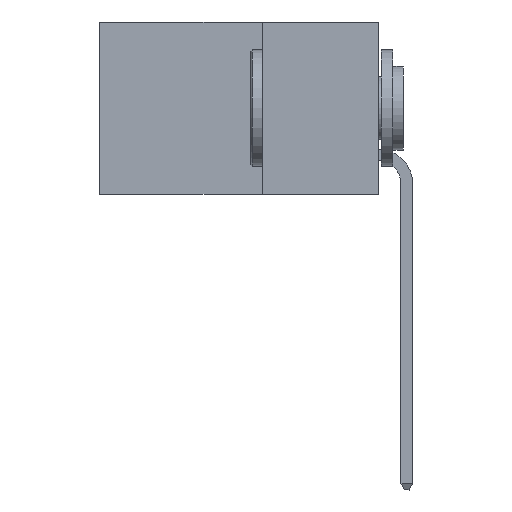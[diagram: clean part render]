
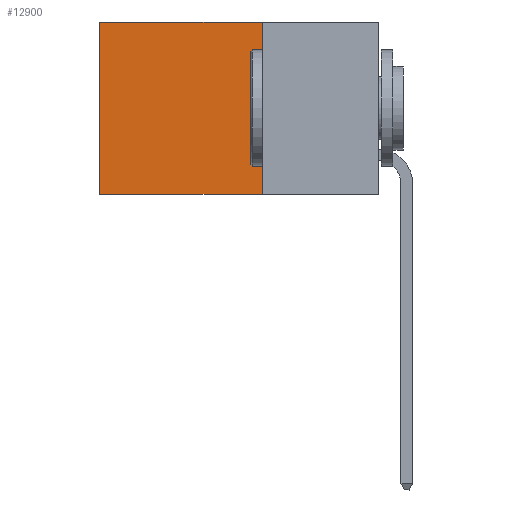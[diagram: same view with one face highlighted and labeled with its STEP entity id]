
A CAD part, left-side view. The second image highlights one B-rep face of the part: STEP entity #12900.
In plain terms, the highlighted planar face has unit normal (-1, 0, 0).
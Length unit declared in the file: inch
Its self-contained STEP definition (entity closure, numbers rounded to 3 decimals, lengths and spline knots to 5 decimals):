
#378 = CARTESIAN_POINT ( 'NONE',  ( 0.2615, 0.25, -0.37 ) ) ;
#1462 = VERTEX_POINT ( 'NONE', #378 ) ;
#1830 = CARTESIAN_POINT ( 'NONE',  ( 0.2615, 0.25, -0.37 ) ) ;
#1868 = DIRECTION ( 'NONE',  ( 0., 1., 0. ) ) ;
#2247 = VERTEX_POINT ( 'NONE', #4230 ) ;
#2530 = VECTOR ( 'NONE', #8465, 39.37008 ) ;
#2884 = AXIS2_PLACEMENT_3D ( 'NONE', #9756, #8778, #9684 ) ;
#3518 = VECTOR ( 'NONE', #1868, 39.37008 ) ;
#3574 = EDGE_LOOP ( 'NONE', ( #5027, #5815, #9888, #6665 ) ) ;
#4083 = LINE ( 'NONE', #1830, #8268 ) ;
#4184 = CARTESIAN_POINT ( 'NONE',  ( 0.2615, 0.25, -0.37 ) ) ;
#4230 = CARTESIAN_POINT ( 'NONE',  ( 0.2615, 0.25, 0. ) ) ;
#4293 = PLANE ( 'NONE',  #2884 ) ;
#5027 = ORIENTED_EDGE ( 'NONE', *, *, #8202, .T. ) ;
#5234 = LINE ( 'NONE', #4184, #2530 ) ;
#5314 = EDGE_CURVE ( 'NONE', #2247, #1462, #5234, .T. ) ;
#5768 = CARTESIAN_POINT ( 'NONE',  ( 0.2615, 0.6, -0.37 ) ) ;
#5794 = VERTEX_POINT ( 'NONE', #12613 ) ;
#5815 = ORIENTED_EDGE ( 'NONE', *, *, #12774, .F. ) ;
#6538 = VERTEX_POINT ( 'NONE', #9650 ) ;
#6665 = ORIENTED_EDGE ( 'NONE', *, *, #9199, .T. ) ;
#6854 = VECTOR ( 'NONE', #13293, 39.37008 ) ;
#8202 = EDGE_CURVE ( 'NONE', #5794, #6538, #11479, .T. ) ;
#8268 = VECTOR ( 'NONE', #10603, 39.37008 ) ;
#8465 = DIRECTION ( 'NONE',  ( 0., 0., -1. ) ) ;
#8778 = DIRECTION ( 'NONE',  ( 1., 0., 0. ) ) ;
#9199 = EDGE_CURVE ( 'NONE', #2247, #5794, #9446, .T. ) ;
#9446 = LINE ( 'NONE', #10508, #3518 ) ;
#9650 = CARTESIAN_POINT ( 'NONE',  ( 0.2615, 0.6, -0.37 ) ) ;
#9684 = DIRECTION ( 'NONE',  ( 0., 0., -1. ) ) ;
#9756 = CARTESIAN_POINT ( 'NONE',  ( 0.2615, 0.25, -0.37 ) ) ;
#9888 = ORIENTED_EDGE ( 'NONE', *, *, #5314, .F. ) ;
#9893 = FACE_OUTER_BOUND ( 'NONE', #3574, .T. ) ;
#10508 = CARTESIAN_POINT ( 'NONE',  ( 0.2615, 0.25, 0. ) ) ;
#10603 = DIRECTION ( 'NONE',  ( 0., 1., 0. ) ) ;
#11479 = LINE ( 'NONE', #5768, #6854 ) ;
#12613 = CARTESIAN_POINT ( 'NONE',  ( 0.2615, 0.6, 0. ) ) ;
#12774 = EDGE_CURVE ( 'NONE', #1462, #6538, #4083, .T. ) ;
#12900 = ADVANCED_FACE ( 'NONE', ( #9893 ), #4293, .F. ) ;
#13293 = DIRECTION ( 'NONE',  ( 0., 0., -1. ) ) ;
